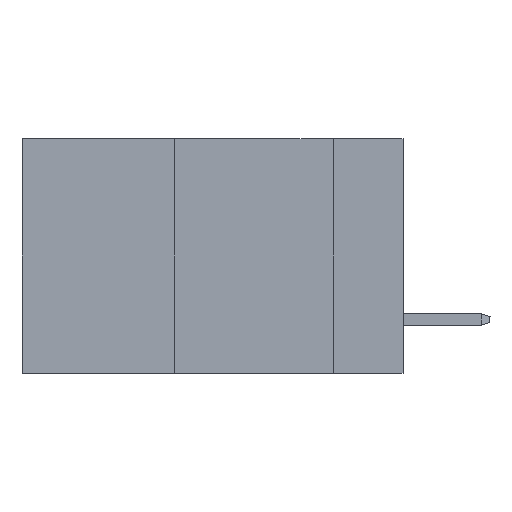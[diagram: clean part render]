
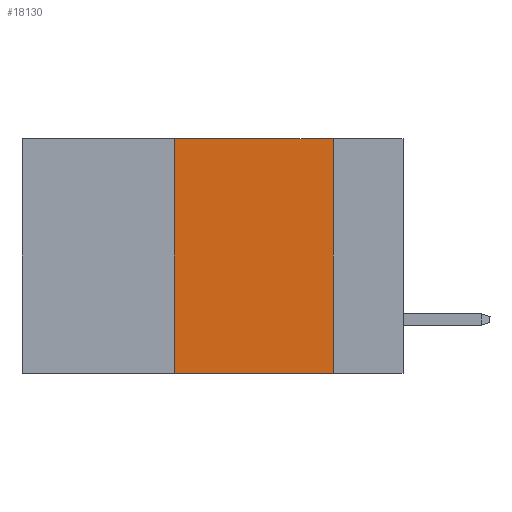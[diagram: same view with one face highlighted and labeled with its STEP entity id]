
A CAD part, left-side view. The second image highlights one B-rep face of the part: STEP entity #18130.
In plain terms, the highlighted planar face has unit normal (-1, 0, 0).
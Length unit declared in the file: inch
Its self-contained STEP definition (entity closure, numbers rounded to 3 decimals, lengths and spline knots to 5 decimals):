
#373 = LINE ( 'NONE', #9391, #3256 ) ;
#1379 = EDGE_CURVE ( 'NONE', #19857, #19693, #1590, .T. ) ;
#1590 = LINE ( 'NONE', #4980, #22546 ) ;
#1990 = LINE ( 'NONE', #2328, #13679 ) ;
#2328 = CARTESIAN_POINT ( 'NONE',  ( 0., 0.11, 0. ) ) ;
#2920 = CARTESIAN_POINT ( 'NONE',  ( 0., 0.11, -0.37 ) ) ;
#3256 = VECTOR ( 'NONE', #14433, 39.37008 ) ;
#3652 = EDGE_CURVE ( 'NONE', #19693, #13112, #373, .T. ) ;
#4063 = CARTESIAN_POINT ( 'NONE',  ( 0., 0.6, -0.37 ) ) ;
#4726 = CARTESIAN_POINT ( 'NONE',  ( 0., 0.36, -0.37 ) ) ;
#4980 = CARTESIAN_POINT ( 'NONE',  ( 0., 0.36, 0. ) ) ;
#7585 = DIRECTION ( 'NONE',  ( 0., -1., 0. ) ) ;
#7648 = CARTESIAN_POINT ( 'NONE',  ( 0., 0.36, 0. ) ) ;
#8151 = PLANE ( 'NONE',  #9523 ) ;
#9391 = CARTESIAN_POINT ( 'NONE',  ( 0., 0.6, 0. ) ) ;
#9523 = AXIS2_PLACEMENT_3D ( 'NONE', #11890, #19127, #12123 ) ;
#10360 = FACE_OUTER_BOUND ( 'NONE', #16813, .T. ) ;
#10826 = ORIENTED_EDGE ( 'NONE', *, *, #1379, .F. ) ;
#11890 = CARTESIAN_POINT ( 'NONE',  ( 0., 0.6, 0. ) ) ;
#12123 = DIRECTION ( 'NONE',  ( 0., 0., -1. ) ) ;
#13112 = VERTEX_POINT ( 'NONE', #18765 ) ;
#13208 = LINE ( 'NONE', #4063, #17691 ) ;
#13679 = VECTOR ( 'NONE', #16250, 39.37008 ) ;
#13792 = ORIENTED_EDGE ( 'NONE', *, *, #3652, .F. ) ;
#14110 = DIRECTION ( 'NONE',  ( 0., 0., 1. ) ) ;
#14433 = DIRECTION ( 'NONE',  ( 0., -1., 0. ) ) ;
#15224 = VERTEX_POINT ( 'NONE', #2920 ) ;
#16250 = DIRECTION ( 'NONE',  ( 0., 0., -1. ) ) ;
#16363 = EDGE_CURVE ( 'NONE', #19857, #15224, #13208, .T. ) ;
#16813 = EDGE_LOOP ( 'NONE', ( #22647, #13792, #10826, #18881 ) ) ;
#17691 = VECTOR ( 'NONE', #7585, 39.37008 ) ;
#18130 = ADVANCED_FACE ( 'NONE', ( #10360 ), #8151, .F. ) ;
#18765 = CARTESIAN_POINT ( 'NONE',  ( 0., 0.11, 0. ) ) ;
#18881 = ORIENTED_EDGE ( 'NONE', *, *, #16363, .T. ) ;
#19127 = DIRECTION ( 'NONE',  ( 1., 0., 0. ) ) ;
#19693 = VERTEX_POINT ( 'NONE', #7648 ) ;
#19857 = VERTEX_POINT ( 'NONE', #4726 ) ;
#21677 = EDGE_CURVE ( 'NONE', #13112, #15224, #1990, .T. ) ;
#22546 = VECTOR ( 'NONE', #14110, 39.37008 ) ;
#22647 = ORIENTED_EDGE ( 'NONE', *, *, #21677, .F. ) ;
